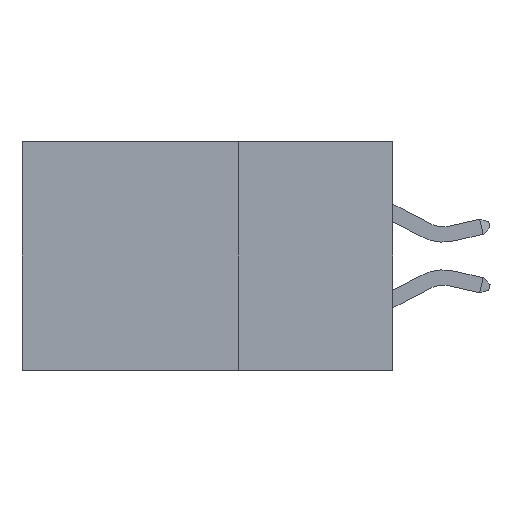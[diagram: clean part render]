
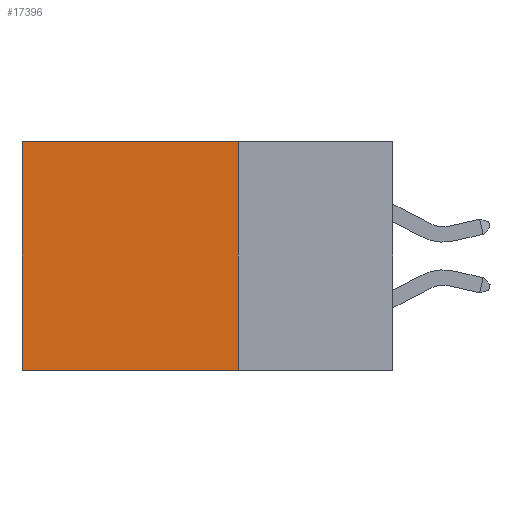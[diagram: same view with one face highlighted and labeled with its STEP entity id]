
A CAD part, left-side view. The second image highlights one B-rep face of the part: STEP entity #17396.
In plain terms, the highlighted planar face has unit normal (-1, 0, 0).
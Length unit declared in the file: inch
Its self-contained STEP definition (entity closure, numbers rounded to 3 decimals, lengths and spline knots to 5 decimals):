
#21 = VECTOR ( 'NONE', #22324, 39.37008 ) ;
#713 = CARTESIAN_POINT ( 'NONE',  ( 0.2875, 0.6, 0. ) ) ;
#1081 = DIRECTION ( 'NONE',  ( 0., 0., -1. ) ) ;
#2135 = VERTEX_POINT ( 'NONE', #9848 ) ;
#2320 = DIRECTION ( 'NONE',  ( 0., 1., 0. ) ) ;
#2439 = PLANE ( 'NONE',  #10306 ) ;
#5246 = DIRECTION ( 'NONE',  ( 0., 1., 0. ) ) ;
#5616 = VECTOR ( 'NONE', #5246, 39.37008 ) ;
#5951 = DIRECTION ( 'NONE',  ( 0., 0., -1. ) ) ;
#6910 = LINE ( 'NONE', #22492, #21 ) ;
#7520 = EDGE_CURVE ( 'NONE', #18465, #2135, #6910, .T. ) ;
#7717 = ORIENTED_EDGE ( 'NONE', *, *, #13470, .T. ) ;
#7848 = FACE_OUTER_BOUND ( 'NONE', #12543, .T. ) ;
#8099 = DIRECTION ( 'NONE',  ( 1., 0., 0. ) ) ;
#9143 = LINE ( 'NONE', #11803, #18682 ) ;
#9523 = ORIENTED_EDGE ( 'NONE', *, *, #12047, .F. ) ;
#9848 = CARTESIAN_POINT ( 'NONE',  ( 0.2875, 0.6, -0.37 ) ) ;
#9906 = ORIENTED_EDGE ( 'NONE', *, *, #17686, .F. ) ;
#10306 = AXIS2_PLACEMENT_3D ( 'NONE', #13502, #8099, #5951 ) ;
#10618 = ORIENTED_EDGE ( 'NONE', *, *, #7520, .T. ) ;
#11803 = CARTESIAN_POINT ( 'NONE',  ( 0.2875, 0.25, 0. ) ) ;
#12047 = EDGE_CURVE ( 'NONE', #14307, #2135, #18416, .T. ) ;
#12543 = EDGE_LOOP ( 'NONE', ( #10618, #9523, #9906, #7717 ) ) ;
#13470 = EDGE_CURVE ( 'NONE', #22577, #18465, #9143, .T. ) ;
#13502 = CARTESIAN_POINT ( 'NONE',  ( 0.2875, 0.25, 0. ) ) ;
#14307 = VERTEX_POINT ( 'NONE', #14397 ) ;
#14397 = CARTESIAN_POINT ( 'NONE',  ( 0.2875, 0.25, -0.37 ) ) ;
#15848 = CARTESIAN_POINT ( 'NONE',  ( 0.2875, 0.25, -0.37 ) ) ;
#17396 = ADVANCED_FACE ( 'NONE', ( #7848 ), #2439, .F. ) ;
#17670 = LINE ( 'NONE', #22131, #19477 ) ;
#17686 = EDGE_CURVE ( 'NONE', #22577, #14307, #17670, .T. ) ;
#18416 = LINE ( 'NONE', #15848, #5616 ) ;
#18465 = VERTEX_POINT ( 'NONE', #713 ) ;
#18682 = VECTOR ( 'NONE', #2320, 39.37008 ) ;
#19477 = VECTOR ( 'NONE', #1081, 39.37008 ) ;
#22131 = CARTESIAN_POINT ( 'NONE',  ( 0.2875, 0.25, 0. ) ) ;
#22324 = DIRECTION ( 'NONE',  ( 0., 0., -1. ) ) ;
#22492 = CARTESIAN_POINT ( 'NONE',  ( 0.2875, 0.6, 0. ) ) ;
#22577 = VERTEX_POINT ( 'NONE', #23847 ) ;
#23847 = CARTESIAN_POINT ( 'NONE',  ( 0.2875, 0.25, 0. ) ) ;
